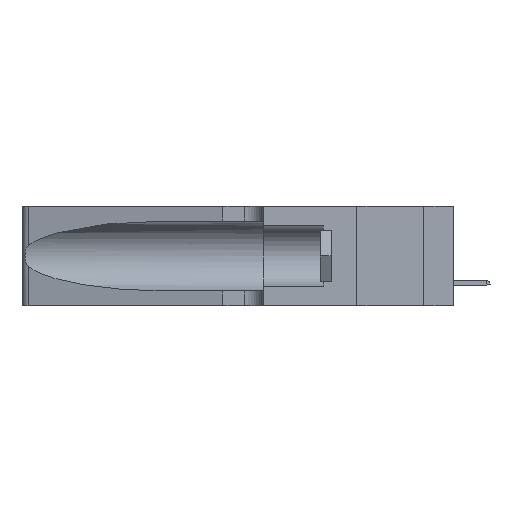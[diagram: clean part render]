
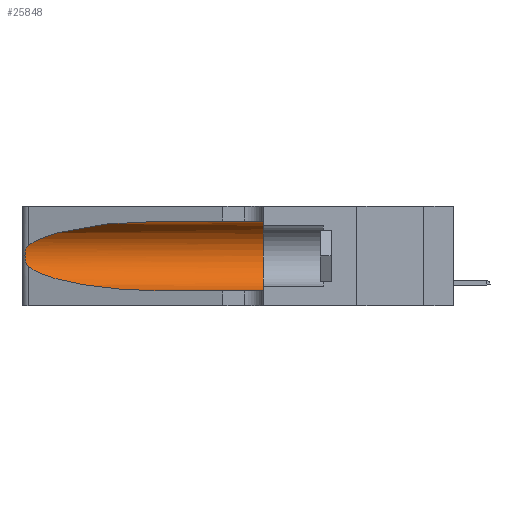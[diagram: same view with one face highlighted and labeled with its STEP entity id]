
A CAD part, left-side view. The second image highlights one B-rep face of the part: STEP entity #25848.
In plain terms, the highlighted cylindrical face has radius 3.308 mm (diameter 6.617 mm), a partial arc.
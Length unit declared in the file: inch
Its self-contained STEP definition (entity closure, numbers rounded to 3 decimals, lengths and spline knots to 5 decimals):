
#450 = VERTEX_POINT ( 'NONE', #32604 ) ;
#876 = DIRECTION ( 'NONE',  ( 0., -1., 0. ) ) ;
#2162 = DIRECTION ( 'NONE',  ( 0., -1., 0. ) ) ;
#2780 = CARTESIAN_POINT ( 'NONE',  ( 0.25487, 1.22718, 0.22369 ) ) ;
#5364 = CARTESIAN_POINT ( 'NONE',  ( 0.25487, 1.22718, 0.14631 ) ) ;
#5418 = CARTESIAN_POINT ( 'NONE',  ( 0.25487, 1.22718, 0.22369 ) ) ;
#5542 = DIRECTION ( 'NONE',  ( 0., 0., -1. ) ) ;
#5966 = AXIS2_PLACEMENT_3D ( 'NONE', #25959, #35189, #16148 ) ;
#7280 = ORIENTED_EDGE ( 'NONE', *, *, #12785, .T. ) ;
#7324 = VERTEX_POINT ( 'NONE', #8693 ) ;
#7983 = ORIENTED_EDGE ( 'NONE', *, *, #31467, .T. ) ;
#8050 = CARTESIAN_POINT ( 'NONE',  ( 0.1305, 0.72297, 0.31525 ) ) ;
#8693 = CARTESIAN_POINT ( 'NONE',  ( 0.1305, 0.35, 0.05475 ) ) ;
#10707 = EDGE_LOOP ( 'NONE', ( #36355, #7280, #7983, #18673, #16246, #29285 ) ) ;
#11321 = CARTESIAN_POINT ( 'NONE',  ( 0.25487, 1.22718, 0.14631 ) ) ;
#11531 = CARTESIAN_POINT ( 'NONE',  ( 0.25639, 1.23184, 0.21858 ) ) ;
#12618 = EDGE_CURVE ( 'NONE', #450, #23775, #25397, .T. ) ;
#12785 = EDGE_CURVE ( 'NONE', #17293, #27406, #24539, .T. ) ;
#14340 = CARTESIAN_POINT ( 'NONE',  ( 0.25555, 1.22994, 0.2215 ) ) ;
#15153 = CARTESIAN_POINT ( 'NONE',  ( 0.25856, 1.23593, 0.16098 ) ) ;
#15391 = CARTESIAN_POINT ( 'NONE',  ( 0.1305, 1.61858, 0.31525 ) ) ;
#15409 = EDGE_CURVE ( 'NONE', #21739, #7324, #21895, .T. ) ;
#15774 = CARTESIAN_POINT ( 'NONE',  ( 0.1305, 0.72297, 0.05475 ) ) ;
#16148 = DIRECTION ( 'NONE',  ( 0., 0., 1. ) ) ;
#16246 = ORIENTED_EDGE ( 'NONE', *, *, #24432, .F. ) ;
#17293 = VERTEX_POINT ( 'NONE', #5418 ) ;
#17518 = AXIS2_PLACEMENT_3D ( 'NONE', #20957, #2162, #5542 ) ;
#18470 = CARTESIAN_POINT ( 'NONE',  ( 0.25555, 1.22993, 0.14849 ) ) ;
#18673 = ORIENTED_EDGE ( 'NONE', *, *, #15409, .T. ) ;
#20637 = CARTESIAN_POINT ( 'NONE',  ( 0.1305, 0.72297, 0.05475 ) ) ;
#20957 = CARTESIAN_POINT ( 'NONE',  ( 0.1305, 1.61858, 0.185 ) ) ;
#21635 = CARTESIAN_POINT ( 'NONE',  ( 0.1305, 0.35, 0.31525 ) ) ;
#21739 = VERTEX_POINT ( 'NONE', #20637 ) ;
#21895 = LINE ( 'NONE', #34310, #34473 ) ;
#21995 = CARTESIAN_POINT ( 'NONE',  ( 0.25487, 1.22718, 0.14631 ) ) ;
#22427 = EDGE_CURVE ( 'NONE', #450, #17293, #22466, .T. ) ;
#22466 =( BOUNDED_CURVE ( )  B_SPLINE_CURVE ( 3, ( #8050, #35116, #25689, #26099 ),
 .UNSPECIFIED., .F., .T. ) 
 B_SPLINE_CURVE_WITH_KNOTS ( ( 4, 4 ),
 ( 1.5708, 2.84003 ),
 .UNSPECIFIED. ) 
 CURVE ( )  GEOMETRIC_REPRESENTATION_ITEM ( )  RATIONAL_B_SPLINE_CURVE ( ( 1., 0.87, 0.87, 1. ) ) 
 REPRESENTATION_ITEM ( '' )  );
#22710 =( BOUNDED_CURVE ( )  B_SPLINE_CURVE ( 3, ( #21995, #24213, #31017, #15774 ),
 .UNSPECIFIED., .F., .F. ) 
 B_SPLINE_CURVE_WITH_KNOTS ( ( 4, 4 ),
 ( 3.44316, 4.71239 ),
 .UNSPECIFIED. ) 
 CURVE ( )  GEOMETRIC_REPRESENTATION_ITEM ( )  RATIONAL_B_SPLINE_CURVE ( ( 1., 0.87, 0.87, 1. ) ) 
 REPRESENTATION_ITEM ( '' )  );
#23775 = VERTEX_POINT ( 'NONE', #21635 ) ;
#23787 = CARTESIAN_POINT ( 'NONE',  ( 0.26075, 1.23896, 0.178 ) ) ;
#24172 = CARTESIAN_POINT ( 'NONE',  ( 0.25854, 1.2359, 0.20912 ) ) ;
#24213 = CARTESIAN_POINT ( 'NONE',  ( 0.2373, 1.15595, 0.08982 ) ) ;
#24432 = EDGE_CURVE ( 'NONE', #23775, #7324, #32186, .T. ) ;
#24539 = B_SPLINE_CURVE_WITH_KNOTS ( 'NONE', 3,
 ( #2780, #14340, #11531, #32816, #24172, #33200, #39409, #23787, #30009, #15153, #27193, #36013, #18470, #5364 ),
 .UNSPECIFIED., .F., .F.,
 ( 4, 2, 2, 2, 2, 2, 4 ),
 ( 0., 0.00027, 0.00053, 0.00107, 0.0016, 0.00187, 0.00214 ),
 .UNSPECIFIED. ) ;
#25397 = LINE ( 'NONE', #15391, #30521 ) ;
#25689 = CARTESIAN_POINT ( 'NONE',  ( 0.2373, 1.15595, 0.28018 ) ) ;
#25848 = ADVANCED_FACE ( 'NONE', ( #36201 ), #38988, .F. ) ;
#25959 = CARTESIAN_POINT ( 'NONE',  ( 0.1305, 0.35, 0.185 ) ) ;
#26099 = CARTESIAN_POINT ( 'NONE',  ( 0.25487, 1.22718, 0.22369 ) ) ;
#27193 = CARTESIAN_POINT ( 'NONE',  ( 0.25789, 1.23486, 0.15765 ) ) ;
#27406 = VERTEX_POINT ( 'NONE', #11321 ) ;
#27647 = DIRECTION ( 'NONE',  ( 0., -1., 0. ) ) ;
#29285 = ORIENTED_EDGE ( 'NONE', *, *, #12618, .F. ) ;
#30009 = CARTESIAN_POINT ( 'NONE',  ( 0.26017, 1.23833, 0.17102 ) ) ;
#30521 = VECTOR ( 'NONE', #27647, 39.37008 ) ;
#31017 = CARTESIAN_POINT ( 'NONE',  ( 0.18966, 0.96281, 0.05475 ) ) ;
#31467 = EDGE_CURVE ( 'NONE', #27406, #21739, #22710, .T. ) ;
#32186 = CIRCLE ( 'NONE', #5966, 0.13025 ) ;
#32604 = CARTESIAN_POINT ( 'NONE',  ( 0.1305, 0.72297, 0.31525 ) ) ;
#32816 = CARTESIAN_POINT ( 'NONE',  ( 0.25787, 1.23484, 0.2124 ) ) ;
#33200 = CARTESIAN_POINT ( 'NONE',  ( 0.26018, 1.23835, 0.19895 ) ) ;
#34310 = CARTESIAN_POINT ( 'NONE',  ( 0.1305, 1.61858, 0.05475 ) ) ;
#34473 = VECTOR ( 'NONE', #876, 39.37008 ) ;
#35116 = CARTESIAN_POINT ( 'NONE',  ( 0.18966, 0.96281, 0.31525 ) ) ;
#35189 = DIRECTION ( 'NONE',  ( 0., 1., 0. ) ) ;
#36013 = CARTESIAN_POINT ( 'NONE',  ( 0.25639, 1.23186, 0.15144 ) ) ;
#36201 = FACE_OUTER_BOUND ( 'NONE', #10707, .T. ) ;
#36355 = ORIENTED_EDGE ( 'NONE', *, *, #22427, .T. ) ;
#38988 = CYLINDRICAL_SURFACE ( 'NONE', #17518, 0.13025 ) ;
#39409 = CARTESIAN_POINT ( 'NONE',  ( 0.26075, 1.23896, 0.19203 ) ) ;
